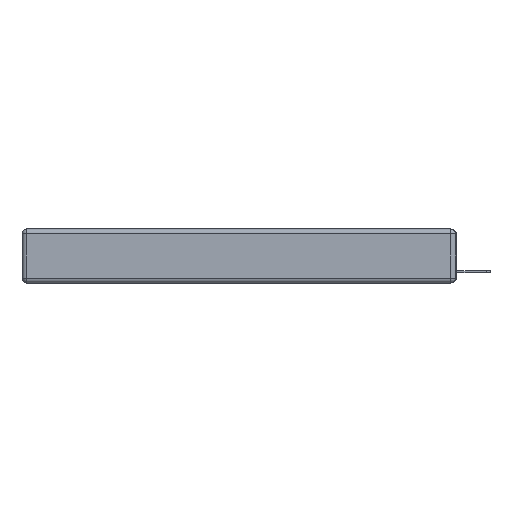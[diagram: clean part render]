
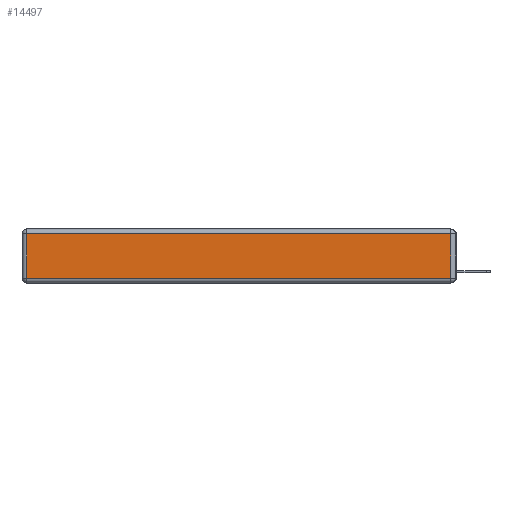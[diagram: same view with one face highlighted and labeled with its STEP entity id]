
A CAD part, left-side view. The second image highlights one B-rep face of the part: STEP entity #14497.
In plain terms, the highlighted planar face has unit normal (-1, 0, 0).
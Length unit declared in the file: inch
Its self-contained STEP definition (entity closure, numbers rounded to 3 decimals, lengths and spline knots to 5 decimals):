
#298 = DIRECTION ( 'NONE',  ( 0., 0., -1. ) ) ;
#1663 = ORIENTED_EDGE ( 'NONE', *, *, #9437, .T. ) ;
#1961 = EDGE_CURVE ( 'NONE', #18926, #6233, #22005, .T. ) ;
#3845 = AXIS2_PLACEMENT_3D ( 'NONE', #9262, #21777, #12808 ) ;
#4441 = LINE ( 'NONE', #20287, #19733 ) ;
#5480 = VECTOR ( 'NONE', #18640, 39.37008 ) ;
#5728 = EDGE_CURVE ( 'NONE', #10208, #19860, #18822, .T. ) ;
#5751 = ORIENTED_EDGE ( 'NONE', *, *, #1961, .T. ) ;
#6039 = CARTESIAN_POINT ( 'NONE',  ( 0., 2.75, -0.03 ) ) ;
#6233 = VERTEX_POINT ( 'NONE', #9568 ) ;
#9262 = CARTESIAN_POINT ( 'NONE',  ( 0., 0., -0.343 ) ) ;
#9437 = EDGE_CURVE ( 'NONE', #6233, #10208, #18515, .T. ) ;
#9568 = CARTESIAN_POINT ( 'NONE',  ( 0., 0.03, -0.313 ) ) ;
#10208 = VERTEX_POINT ( 'NONE', #12170 ) ;
#11079 = EDGE_CURVE ( 'NONE', #19860, #18926, #4441, .T. ) ;
#11137 = VECTOR ( 'NONE', #22169, 39.37008 ) ;
#11148 = PLANE ( 'NONE',  #3845 ) ;
#11884 = EDGE_LOOP ( 'NONE', ( #5751, #1663, #15523, #12413 ) ) ;
#12170 = CARTESIAN_POINT ( 'NONE',  ( 0., 0.03, -0.03 ) ) ;
#12413 = ORIENTED_EDGE ( 'NONE', *, *, #11079, .T. ) ;
#12808 = DIRECTION ( 'NONE',  ( 0., 0., 1. ) ) ;
#12820 = CARTESIAN_POINT ( 'NONE',  ( 0., 2.72, -0.03 ) ) ;
#14072 = VECTOR ( 'NONE', #17899, 39.37008 ) ;
#14497 = ADVANCED_FACE ( 'NONE', ( #17413 ), #11148, .T. ) ;
#15523 = ORIENTED_EDGE ( 'NONE', *, *, #5728, .T. ) ;
#17413 = FACE_OUTER_BOUND ( 'NONE', #11884, .T. ) ;
#17899 = DIRECTION ( 'NONE',  ( 0., -1., 0. ) ) ;
#18515 = LINE ( 'NONE', #20397, #5480 ) ;
#18640 = DIRECTION ( 'NONE',  ( 0., 0., 1. ) ) ;
#18822 = LINE ( 'NONE', #6039, #11137 ) ;
#18926 = VERTEX_POINT ( 'NONE', #20052 ) ;
#19733 = VECTOR ( 'NONE', #298, 39.37008 ) ;
#19860 = VERTEX_POINT ( 'NONE', #12820 ) ;
#20052 = CARTESIAN_POINT ( 'NONE',  ( 0., 2.72, -0.313 ) ) ;
#20287 = CARTESIAN_POINT ( 'NONE',  ( 0., 2.72, -0.343 ) ) ;
#20397 = CARTESIAN_POINT ( 'NONE',  ( 0., 0.03, -0.343 ) ) ;
#21752 = CARTESIAN_POINT ( 'NONE',  ( 0., 0., -0.313 ) ) ;
#21777 = DIRECTION ( 'NONE',  ( -1., 0., 0. ) ) ;
#22005 = LINE ( 'NONE', #21752, #14072 ) ;
#22169 = DIRECTION ( 'NONE',  ( 0., 1., 0. ) ) ;
